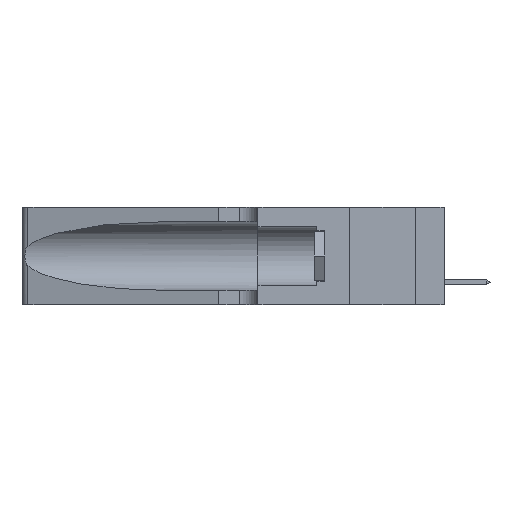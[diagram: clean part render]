
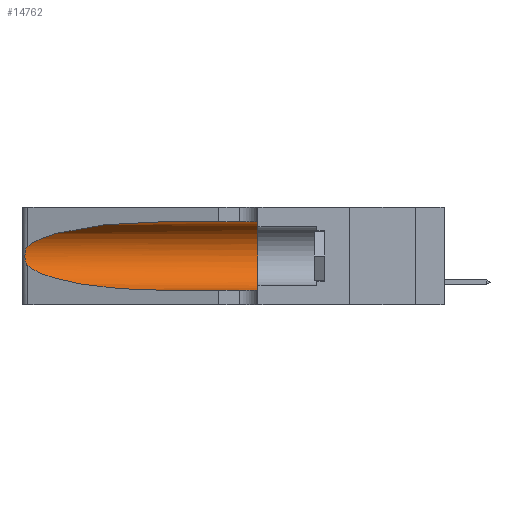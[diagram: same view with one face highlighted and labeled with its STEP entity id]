
A CAD part, left-side view. The second image highlights one B-rep face of the part: STEP entity #14762.
In plain terms, the highlighted cylindrical face has radius 3.308 mm (diameter 6.617 mm), a partial arc.
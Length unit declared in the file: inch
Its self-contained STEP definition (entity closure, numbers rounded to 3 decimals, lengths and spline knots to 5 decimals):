
#1015 = FACE_OUTER_BOUND ( 'NONE', #3768, .T. ) ;
#1242 = CARTESIAN_POINT ( 'NONE',  ( 0.25487, 1.22718, 0.14631 ) ) ;
#1352 = CARTESIAN_POINT ( 'NONE',  ( 0.26075, 1.23896, 0.19203 ) ) ;
#1469 = CARTESIAN_POINT ( 'NONE',  ( 0.25639, 1.23184, 0.21858 ) ) ;
#1622 = VECTOR ( 'NONE', #28251, 39.37008 ) ;
#1760 = CARTESIAN_POINT ( 'NONE',  ( 0.25487, 1.22718, 0.22369 ) ) ;
#3006 = ORIENTED_EDGE ( 'NONE', *, *, #10235, .T. ) ;
#3116 = ORIENTED_EDGE ( 'NONE', *, *, #7700, .F. ) ;
#3768 = EDGE_LOOP ( 'NONE', ( #19162, #7542, #5114, #3006, #3116, #10218 ) ) ;
#4037 = DIRECTION ( 'NONE',  ( 0., 0., 1. ) ) ;
#5049 = EDGE_CURVE ( 'NONE', #16157, #19617, #12208, .T. ) ;
#5114 = ORIENTED_EDGE ( 'NONE', *, *, #5049, .T. ) ;
#5225 = LINE ( 'NONE', #20000, #1622 ) ;
#6355 = CARTESIAN_POINT ( 'NONE',  ( 0.25789, 1.23486, 0.15765 ) ) ;
#6780 = B_SPLINE_CURVE_WITH_KNOTS ( 'NONE', 3,
 ( #26483, #11533, #1469, #13758, #31441, #24267, #1352, #29241, #18963, #9089, #6355, #14084, #19074, #1242 ),
 .UNSPECIFIED., .F., .F.,
 ( 4, 2, 2, 2, 2, 2, 4 ),
 ( 0., 0.00027, 0.00053, 0.00107, 0.0016, 0.00187, 0.00214 ),
 .UNSPECIFIED. ) ;
#6947 = CARTESIAN_POINT ( 'NONE',  ( 0.25487, 1.22718, 0.22369 ) ) ;
#7542 = ORIENTED_EDGE ( 'NONE', *, *, #32089, .T. ) ;
#7700 = EDGE_CURVE ( 'NONE', #28497, #14466, #30389, .T. ) ;
#7886 = DIRECTION ( 'NONE',  ( 0., -1., 0. ) ) ;
#9089 = CARTESIAN_POINT ( 'NONE',  ( 0.25856, 1.23593, 0.16098 ) ) ;
#9712 = CARTESIAN_POINT ( 'NONE',  ( 0.1305, 0.72297, 0.05475 ) ) ;
#10168 = CARTESIAN_POINT ( 'NONE',  ( 0.18966, 0.96281, 0.05475 ) ) ;
#10218 = ORIENTED_EDGE ( 'NONE', *, *, #10716, .F. ) ;
#10235 = EDGE_CURVE ( 'NONE', #19617, #14466, #30170, .T. ) ;
#10716 = EDGE_CURVE ( 'NONE', #24121, #28497, #5225, .T. ) ;
#11533 = CARTESIAN_POINT ( 'NONE',  ( 0.25555, 1.22994, 0.2215 ) ) ;
#11908 = CARTESIAN_POINT ( 'NONE',  ( 0.2373, 1.15595, 0.28018 ) ) ;
#12208 =( BOUNDED_CURVE ( )  B_SPLINE_CURVE ( 3, ( #20176, #23010, #10168, #27543 ),
 .UNSPECIFIED., .F., .F. ) 
 B_SPLINE_CURVE_WITH_KNOTS ( ( 4, 4 ),
 ( 3.44316, 4.71239 ),
 .UNSPECIFIED. ) 
 CURVE ( )  GEOMETRIC_REPRESENTATION_ITEM ( )  RATIONAL_B_SPLINE_CURVE ( ( 1., 0.87, 0.87, 1. ) ) 
 REPRESENTATION_ITEM ( '' )  );
#13758 = CARTESIAN_POINT ( 'NONE',  ( 0.25787, 1.23484, 0.2124 ) ) ;
#14084 = CARTESIAN_POINT ( 'NONE',  ( 0.25639, 1.23186, 0.15144 ) ) ;
#14466 = VERTEX_POINT ( 'NONE', #30733 ) ;
#14562 = CARTESIAN_POINT ( 'NONE',  ( 0.18966, 0.96281, 0.31525 ) ) ;
#14762 = ADVANCED_FACE ( 'NONE', ( #1015 ), #22037, .F. ) ;
#14866 = CARTESIAN_POINT ( 'NONE',  ( 0.1305, 0.72297, 0.31525 ) ) ;
#16157 = VERTEX_POINT ( 'NONE', #23738 ) ;
#16623 = DIRECTION ( 'NONE',  ( 0., 1., 0. ) ) ;
#16638 = CARTESIAN_POINT ( 'NONE',  ( 0.1305, 0.35, 0.31525 ) ) ;
#18040 = DIRECTION ( 'NONE',  ( 0., 0., -1. ) ) ;
#18963 = CARTESIAN_POINT ( 'NONE',  ( 0.26017, 1.23833, 0.17102 ) ) ;
#19074 = CARTESIAN_POINT ( 'NONE',  ( 0.25555, 1.22993, 0.14849 ) ) ;
#19108 = VERTEX_POINT ( 'NONE', #1760 ) ;
#19162 = ORIENTED_EDGE ( 'NONE', *, *, #20485, .T. ) ;
#19239 = DIRECTION ( 'NONE',  ( 0., -1., 0. ) ) ;
#19617 = VERTEX_POINT ( 'NONE', #9712 ) ;
#20000 = CARTESIAN_POINT ( 'NONE',  ( 0.1305, 1.61858, 0.31525 ) ) ;
#20176 = CARTESIAN_POINT ( 'NONE',  ( 0.25487, 1.22718, 0.14631 ) ) ;
#20485 = EDGE_CURVE ( 'NONE', #24121, #19108, #27418, .T. ) ;
#20585 = CARTESIAN_POINT ( 'NONE',  ( 0.1305, 1.61858, 0.185 ) ) ;
#21462 = CARTESIAN_POINT ( 'NONE',  ( 0.1305, 1.61858, 0.05475 ) ) ;
#22037 = CYLINDRICAL_SURFACE ( 'NONE', #27654, 0.13025 ) ;
#22793 = CARTESIAN_POINT ( 'NONE',  ( 0.1305, 0.72297, 0.31525 ) ) ;
#23010 = CARTESIAN_POINT ( 'NONE',  ( 0.2373, 1.15595, 0.08982 ) ) ;
#23738 = CARTESIAN_POINT ( 'NONE',  ( 0.25487, 1.22718, 0.14631 ) ) ;
#24121 = VERTEX_POINT ( 'NONE', #22793 ) ;
#24267 = CARTESIAN_POINT ( 'NONE',  ( 0.26018, 1.23835, 0.19895 ) ) ;
#26483 = CARTESIAN_POINT ( 'NONE',  ( 0.25487, 1.22718, 0.22369 ) ) ;
#27418 =( BOUNDED_CURVE ( )  B_SPLINE_CURVE ( 3, ( #14866, #14562, #11908, #6947 ),
 .UNSPECIFIED., .F., .T. ) 
 B_SPLINE_CURVE_WITH_KNOTS ( ( 4, 4 ),
 ( 1.5708, 2.84003 ),
 .UNSPECIFIED. ) 
 CURVE ( )  GEOMETRIC_REPRESENTATION_ITEM ( )  RATIONAL_B_SPLINE_CURVE ( ( 1., 0.87, 0.87, 1. ) ) 
 REPRESENTATION_ITEM ( '' )  );
#27543 = CARTESIAN_POINT ( 'NONE',  ( 0.1305, 0.72297, 0.05475 ) ) ;
#27654 = AXIS2_PLACEMENT_3D ( 'NONE', #20585, #7886, #18040 ) ;
#28251 = DIRECTION ( 'NONE',  ( 0., -1., 0. ) ) ;
#28497 = VERTEX_POINT ( 'NONE', #16638 ) ;
#28988 = VECTOR ( 'NONE', #19239, 39.37008 ) ;
#29241 = CARTESIAN_POINT ( 'NONE',  ( 0.26075, 1.23896, 0.178 ) ) ;
#29243 = CARTESIAN_POINT ( 'NONE',  ( 0.1305, 0.35, 0.185 ) ) ;
#30038 = AXIS2_PLACEMENT_3D ( 'NONE', #29243, #16623, #4037 ) ;
#30170 = LINE ( 'NONE', #21462, #28988 ) ;
#30389 = CIRCLE ( 'NONE', #30038, 0.13025 ) ;
#30733 = CARTESIAN_POINT ( 'NONE',  ( 0.1305, 0.35, 0.05475 ) ) ;
#31441 = CARTESIAN_POINT ( 'NONE',  ( 0.25854, 1.2359, 0.20912 ) ) ;
#32089 = EDGE_CURVE ( 'NONE', #19108, #16157, #6780, .T. ) ;
